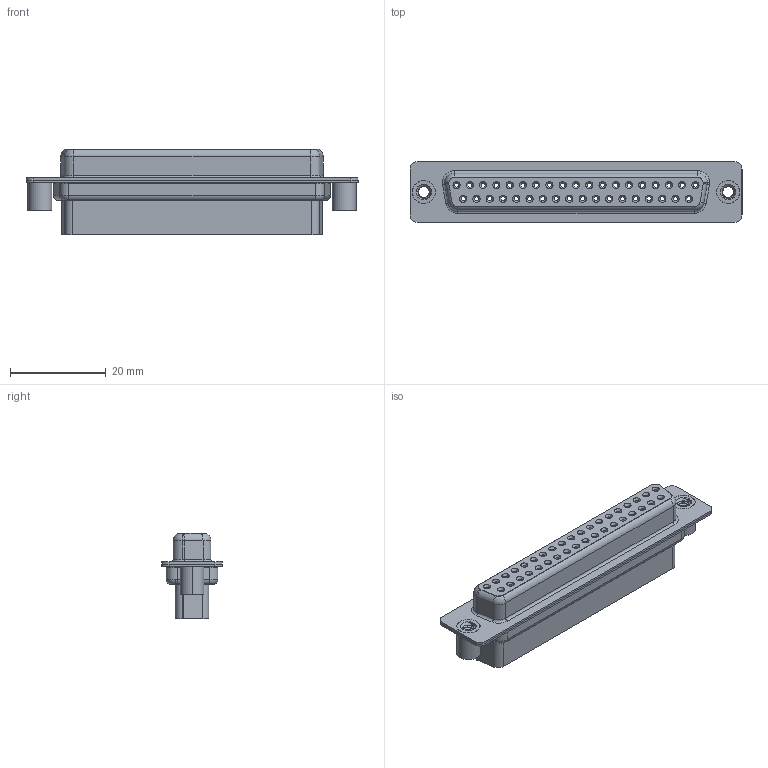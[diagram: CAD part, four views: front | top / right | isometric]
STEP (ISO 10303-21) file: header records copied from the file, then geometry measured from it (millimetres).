
FILE_DESCRIPTION (( 'STEP AP203' ), '1' );
FILE_NAME ('628-050-010-220.STEP', '2018-11-21T22:15:18', ( '' ), ( '' ), 'SwSTEP 2.0', 'SolidWorks 2016', '' );
FILE_SCHEMA (( 'CONFIG_CONTROL_DESIGN' ));
Length unit declared in the file: millimetre
Products named in the file (5): 628 Shell Rear_37 Contacts; 628 4-40 Threaded Standoff BS; 628-050-010-220; 628 Housing_37 HP; 628 Shell Front_37 Contacts
Assembly tree (5 placements, depth 2):
  628-050-010-220
    628 Housing_37 HP
    628 Shell Front_37 Contacts
    628 Shell Rear_37 Contacts
    628 4-40 Threaded Standoff BS  x2
Bounding box: 69.3 x 12.6 x 17.9 mm (x, y, z)
Volume: 6760.7 mm3; surface area: 11143.8 mm2
Topology: 5 solids, 5 shells, 782 faces, 1785 edges, 1135 vertices
Faces by surface type: cylinder 453, plane 178, cone 88, torus 57, bspline 6
Entity records: 23330 total; most frequent: CARTESIAN_POINT 5388, DIRECTION 4007, ORIENTED_EDGE 3344, AXIS2_PLACEMENT_3D 1689, EDGE_CURVE 1672, VERTEX_POINT 1062, CIRCLE 946, EDGE_LOOP 946
